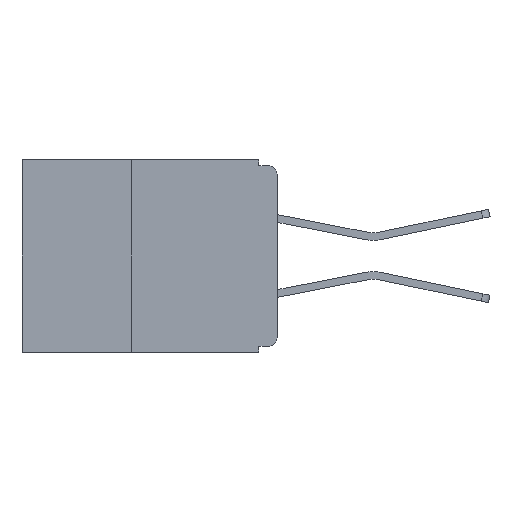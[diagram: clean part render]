
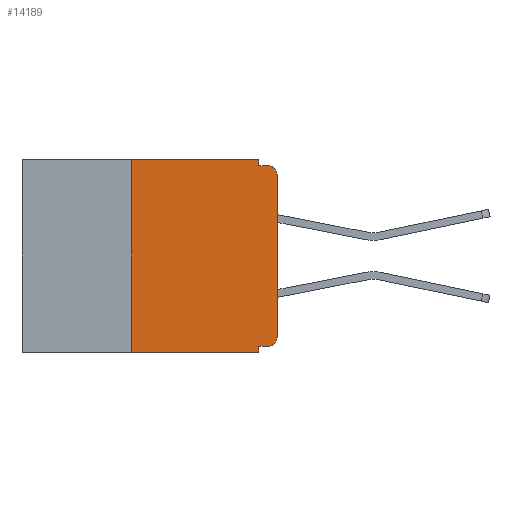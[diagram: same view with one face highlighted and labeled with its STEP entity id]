
A CAD part, left-side view. The second image highlights one B-rep face of the part: STEP entity #14189.
In plain terms, the highlighted planar face has unit normal (-1, 0, 0).
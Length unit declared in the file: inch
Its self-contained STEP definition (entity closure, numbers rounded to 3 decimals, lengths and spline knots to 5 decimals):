
#762 = DIRECTION ( 'NONE',  ( 0., -1., 0. ) ) ;
#832 = EDGE_CURVE ( 'NONE', #17733, #6788, #8148, .T. ) ;
#984 = VERTEX_POINT ( 'NONE', #30475 ) ;
#1595 = VECTOR ( 'NONE', #19309, 39.37008 ) ;
#1703 = VERTEX_POINT ( 'NONE', #16572 ) ;
#1949 = EDGE_CURVE ( 'NONE', #6788, #984, #20798, .T. ) ;
#1998 = DIRECTION ( 'NONE',  ( 1., 0., 0. ) ) ;
#2247 = LINE ( 'NONE', #4406, #26737 ) ;
#2268 = EDGE_CURVE ( 'NONE', #12545, #8203, #19547, .T. ) ;
#2449 = EDGE_CURVE ( 'NONE', #984, #8055, #7966, .T. ) ;
#4062 = ORIENTED_EDGE ( 'NONE', *, *, #29923, .T. ) ;
#4406 = CARTESIAN_POINT ( 'NONE',  ( 0., 0., -0.01 ) ) ;
#4877 = VECTOR ( 'NONE', #5178, 39.37008 ) ;
#5178 = DIRECTION ( 'NONE',  ( 0., -1., 0. ) ) ;
#5805 = AXIS2_PLACEMENT_3D ( 'NONE', #9415, #26012, #11861 ) ;
#6349 = EDGE_LOOP ( 'NONE', ( #13401, #8511, #27399, #28106, #11537, #8160, #4062, #16792, #7065, #14917 ) ) ;
#6788 = VERTEX_POINT ( 'NONE', #15931 ) ;
#6853 = VECTOR ( 'NONE', #18493, 39.37008 ) ;
#6891 = AXIS2_PLACEMENT_3D ( 'NONE', #14183, #30519, #16571 ) ;
#7065 = ORIENTED_EDGE ( 'NONE', *, *, #2268, .F. ) ;
#7313 = LINE ( 'NONE', #27717, #12944 ) ;
#7966 = LINE ( 'NONE', #16944, #1595 ) ;
#8055 = VERTEX_POINT ( 'NONE', #21781 ) ;
#8122 = VECTOR ( 'NONE', #762, 39.37008 ) ;
#8148 = LINE ( 'NONE', #22507, #20084 ) ;
#8160 = ORIENTED_EDGE ( 'NONE', *, *, #832, .F. ) ;
#8203 = VERTEX_POINT ( 'NONE', #15118 ) ;
#8511 = ORIENTED_EDGE ( 'NONE', *, *, #29754, .T. ) ;
#9415 = CARTESIAN_POINT ( 'NONE',  ( 0., 0.015, -0.305 ) ) ;
#9469 = VERTEX_POINT ( 'NONE', #10639 ) ;
#10639 = CARTESIAN_POINT ( 'NONE',  ( 0., 0.031, -0.33 ) ) ;
#11537 = ORIENTED_EDGE ( 'NONE', *, *, #1949, .F. ) ;
#11861 = DIRECTION ( 'NONE',  ( 0., 0., -1. ) ) ;
#11894 = EDGE_CURVE ( 'NONE', #8055, #1703, #2247, .T. ) ;
#12545 = VERTEX_POINT ( 'NONE', #21043 ) ;
#12705 = LINE ( 'NONE', #30249, #24566 ) ;
#12944 = VECTOR ( 'NONE', #29990, 39.37008 ) ;
#13401 = ORIENTED_EDGE ( 'NONE', *, *, #19841, .T. ) ;
#13901 = DIRECTION ( 'NONE',  ( 0., 0., 1. ) ) ;
#13938 = PLANE ( 'NONE',  #30550 ) ;
#14183 = CARTESIAN_POINT ( 'NONE',  ( 0., 0.015, -0.025 ) ) ;
#14189 = ADVANCED_FACE ( 'NONE', ( #24858 ), #13938, .F. ) ;
#14917 = ORIENTED_EDGE ( 'NONE', *, *, #25154, .T. ) ;
#15088 = CARTESIAN_POINT ( 'NONE',  ( 0., 0.437, 0. ) ) ;
#15118 = CARTESIAN_POINT ( 'NONE',  ( 0., 0.031, -0.32 ) ) ;
#15931 = CARTESIAN_POINT ( 'NONE',  ( 0., 0.25, 0. ) ) ;
#16311 = CIRCLE ( 'NONE', #5805, 0.015 ) ;
#16467 = CIRCLE ( 'NONE', #6891, 0.015 ) ;
#16571 = DIRECTION ( 'NONE',  ( 0., 0., -1. ) ) ;
#16572 = CARTESIAN_POINT ( 'NONE',  ( 0., 0.015, -0.01 ) ) ;
#16792 = ORIENTED_EDGE ( 'NONE', *, *, #26882, .F. ) ;
#16944 = CARTESIAN_POINT ( 'NONE',  ( 0., 0.031, 0. ) ) ;
#17733 = VERTEX_POINT ( 'NONE', #18131 ) ;
#18131 = CARTESIAN_POINT ( 'NONE',  ( 0., 0.25, -0.33 ) ) ;
#18493 = DIRECTION ( 'NONE',  ( 0., 1., 0. ) ) ;
#18597 = CARTESIAN_POINT ( 'NONE',  ( 0., 0., -0.32 ) ) ;
#18695 = DIRECTION ( 'NONE',  ( 0., 0., -1. ) ) ;
#19309 = DIRECTION ( 'NONE',  ( 0., 0., -1. ) ) ;
#19547 = LINE ( 'NONE', #18597, #6853 ) ;
#19841 = EDGE_CURVE ( 'NONE', #28974, #22899, #12705, .T. ) ;
#20084 = VECTOR ( 'NONE', #22432, 39.37008 ) ;
#20529 = CARTESIAN_POINT ( 'NONE',  ( 0., 0., -0.305 ) ) ;
#20798 = LINE ( 'NONE', #15088, #8122 ) ;
#20847 = CARTESIAN_POINT ( 'NONE',  ( 0., 0., -0.025 ) ) ;
#21043 = CARTESIAN_POINT ( 'NONE',  ( 0., 0.015, -0.32 ) ) ;
#21781 = CARTESIAN_POINT ( 'NONE',  ( 0., 0.031, -0.01 ) ) ;
#22432 = DIRECTION ( 'NONE',  ( 0., 0., 1. ) ) ;
#22507 = CARTESIAN_POINT ( 'NONE',  ( 0., 0.25, -0.33 ) ) ;
#22899 = VERTEX_POINT ( 'NONE', #20847 ) ;
#24566 = VECTOR ( 'NONE', #13901, 39.37008 ) ;
#24858 = FACE_OUTER_BOUND ( 'NONE', #6349, .T. ) ;
#25154 = EDGE_CURVE ( 'NONE', #12545, #28974, #16311, .T. ) ;
#25783 = DIRECTION ( 'NONE',  ( 0., -1., 0. ) ) ;
#26012 = DIRECTION ( 'NONE',  ( -1., 0., 0. ) ) ;
#26511 = CARTESIAN_POINT ( 'NONE',  ( 0., 0.437, -0.33 ) ) ;
#26737 = VECTOR ( 'NONE', #25783, 39.37008 ) ;
#26882 = EDGE_CURVE ( 'NONE', #8203, #9469, #7313, .T. ) ;
#27399 = ORIENTED_EDGE ( 'NONE', *, *, #11894, .F. ) ;
#27717 = CARTESIAN_POINT ( 'NONE',  ( 0., 0.031, -0.33 ) ) ;
#28106 = ORIENTED_EDGE ( 'NONE', *, *, #2449, .F. ) ;
#28974 = VERTEX_POINT ( 'NONE', #20529 ) ;
#29754 = EDGE_CURVE ( 'NONE', #22899, #1703, #16467, .T. ) ;
#29923 = EDGE_CURVE ( 'NONE', #17733, #9469, #29936, .T. ) ;
#29936 = LINE ( 'NONE', #26511, #4877 ) ;
#29990 = DIRECTION ( 'NONE',  ( 0., 0., -1. ) ) ;
#30249 = CARTESIAN_POINT ( 'NONE',  ( 0., 0., 0. ) ) ;
#30283 = CARTESIAN_POINT ( 'NONE',  ( 0., 0.437, 0. ) ) ;
#30475 = CARTESIAN_POINT ( 'NONE',  ( 0., 0.031, 0. ) ) ;
#30519 = DIRECTION ( 'NONE',  ( -1., 0., 0. ) ) ;
#30550 = AXIS2_PLACEMENT_3D ( 'NONE', #30283, #1998, #18695 ) ;
